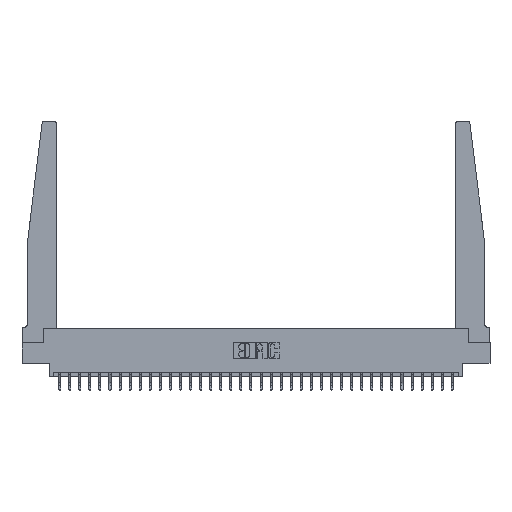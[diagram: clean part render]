
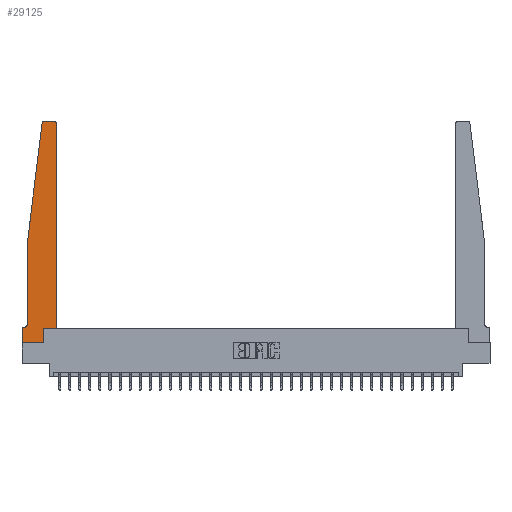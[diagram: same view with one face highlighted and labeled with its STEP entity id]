
A CAD part, top view. The second image highlights one B-rep face of the part: STEP entity #29125.
In plain terms, the highlighted planar face has unit normal (0, 0, 1).
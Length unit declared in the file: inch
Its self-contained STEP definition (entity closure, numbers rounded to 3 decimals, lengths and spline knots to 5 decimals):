
#101 = VERTEX_POINT ( 'NONE', #22427 ) ;
#402 = VERTEX_POINT ( 'NONE', #6686 ) ;
#504 = ORIENTED_EDGE ( 'NONE', *, *, #11489, .T. ) ;
#626 = VERTEX_POINT ( 'NONE', #10877 ) ;
#701 = AXIS2_PLACEMENT_3D ( 'NONE', #30100, #7908, #3069 ) ;
#1510 = DIRECTION ( 'NONE',  ( 1., 0., 0. ) ) ;
#1739 = DIRECTION ( 'NONE',  ( -1., 0., 0. ) ) ;
#1906 = LINE ( 'NONE', #29407, #7983 ) ;
#1941 = VERTEX_POINT ( 'NONE', #22807 ) ;
#2016 = AXIS2_PLACEMENT_3D ( 'NONE', #30453, #7793, #10555 ) ;
#2256 = EDGE_CURVE ( 'NONE', #402, #26183, #29090, .T. ) ;
#2539 = EDGE_CURVE ( 'NONE', #26183, #1941, #19875, .T. ) ;
#3069 = DIRECTION ( 'NONE',  ( -1., 0., 0. ) ) ;
#3505 = CARTESIAN_POINT ( 'NONE',  ( 0.2605, 0.18, 0.37 ) ) ;
#3759 = CARTESIAN_POINT ( 'NONE',  ( 0., 0., 0.37 ) ) ;
#3989 = ORIENTED_EDGE ( 'NONE', *, *, #30733, .T. ) ;
#4038 = ORIENTED_EDGE ( 'NONE', *, *, #2539, .T. ) ;
#4169 = VERTEX_POINT ( 'NONE', #20301 ) ;
#4777 = CARTESIAN_POINT ( 'NONE',  ( 0., 0., 0.37 ) ) ;
#5580 = ORIENTED_EDGE ( 'NONE', *, *, #31310, .T. ) ;
#5649 = LINE ( 'NONE', #10828, #10124 ) ;
#5750 = DIRECTION ( 'NONE',  ( 0., 0., 1. ) ) ;
#6127 = ORIENTED_EDGE ( 'NONE', *, *, #16061, .T. ) ;
#6518 = LINE ( 'NONE', #3759, #27397 ) ;
#6686 = CARTESIAN_POINT ( 'NONE',  ( 0.395, 2.75, 0.37 ) ) ;
#7451 = EDGE_CURVE ( 'NONE', #31533, #101, #13365, .T. ) ;
#7793 = DIRECTION ( 'NONE',  ( 0., 0., 1. ) ) ;
#7827 = FACE_OUTER_BOUND ( 'NONE', #25704, .T. ) ;
#7892 = CARTESIAN_POINT ( 'NONE',  ( 0.2605, 0., 0.37 ) ) ;
#7908 = DIRECTION ( 'NONE',  ( 0., 0., -1. ) ) ;
#7983 = VECTOR ( 'NONE', #11783, 39.37008 ) ;
#8486 = AXIS2_PLACEMENT_3D ( 'NONE', #18069, #5750, #23089 ) ;
#8631 = ORIENTED_EDGE ( 'NONE', *, *, #29438, .T. ) ;
#8646 = VECTOR ( 'NONE', #24227, 39.37008 ) ;
#9258 = AXIS2_PLACEMENT_3D ( 'NONE', #18044, #22742, #20772 ) ;
#9527 = VECTOR ( 'NONE', #17424, 39.37008 ) ;
#9723 = LINE ( 'NONE', #9867, #14755 ) ;
#9867 = CARTESIAN_POINT ( 'NONE',  ( 0.065, 1.25, 0.37 ) ) ;
#10124 = VECTOR ( 'NONE', #15526, 39.37008 ) ;
#10555 = DIRECTION ( 'NONE',  ( 1., 0., 0. ) ) ;
#10763 = ORIENTED_EDGE ( 'NONE', *, *, #12258, .T. ) ;
#10828 = CARTESIAN_POINT ( 'NONE',  ( 0.065, 0.1875, 0.37 ) ) ;
#10877 = CARTESIAN_POINT ( 'NONE',  ( 0., 0., 0.37 ) ) ;
#11275 = CARTESIAN_POINT ( 'NONE',  ( 0.065, 0.2375, 0.37 ) ) ;
#11489 = EDGE_CURVE ( 'NONE', #12859, #12520, #1906, .T. ) ;
#11535 = DIRECTION ( 'NONE',  ( 0., -1., 0. ) ) ;
#11783 = DIRECTION ( 'NONE',  ( 0., 1., 0. ) ) ;
#12258 = EDGE_CURVE ( 'NONE', #14881, #27483, #9723, .T. ) ;
#12520 = VERTEX_POINT ( 'NONE', #29776 ) ;
#12859 = VERTEX_POINT ( 'NONE', #26493 ) ;
#12861 = PLANE ( 'NONE',  #9258 ) ;
#13365 = LINE ( 'NONE', #3505, #21335 ) ;
#14755 = VECTOR ( 'NONE', #11535, 39.37008 ) ;
#14832 = LINE ( 'NONE', #16768, #8646 ) ;
#14881 = VERTEX_POINT ( 'NONE', #19073 ) ;
#15020 = VERTEX_POINT ( 'NONE', #23779 ) ;
#15302 = VECTOR ( 'NONE', #1739, 39.37008 ) ;
#15526 = DIRECTION ( 'NONE',  ( -1., 0., 0. ) ) ;
#16061 = EDGE_CURVE ( 'NONE', #27483, #4169, #21400, .T. ) ;
#16768 = CARTESIAN_POINT ( 'NONE',  ( 0.065, 1.25, 0.37 ) ) ;
#16770 = EDGE_CURVE ( 'NONE', #15020, #626, #31631, .T. ) ;
#17424 = DIRECTION ( 'NONE',  ( 0., -1., 0. ) ) ;
#17673 = ORIENTED_EDGE ( 'NONE', *, *, #7451, .T. ) ;
#18044 = CARTESIAN_POINT ( 'NONE',  ( 0., 0.1875, 0.37 ) ) ;
#18069 = CARTESIAN_POINT ( 'NONE',  ( 0.27653, 2.72, 0.37 ) ) ;
#18947 = CARTESIAN_POINT ( 'NONE',  ( 0.425, 0.18, 0.37 ) ) ;
#19073 = CARTESIAN_POINT ( 'NONE',  ( 0.065, 1.25, 0.37 ) ) ;
#19875 = CIRCLE ( 'NONE', #8486, 0.03 ) ;
#20205 = VECTOR ( 'NONE', #29302, 39.37008 ) ;
#20301 = CARTESIAN_POINT ( 'NONE',  ( 0.015, 0.1875, 0.37 ) ) ;
#20772 = DIRECTION ( 'NONE',  ( 1., 0., 0. ) ) ;
#21335 = VECTOR ( 'NONE', #23258, 39.37008 ) ;
#21400 = CIRCLE ( 'NONE', #701, 0.05 ) ;
#22427 = CARTESIAN_POINT ( 'NONE',  ( 0.2605, 0.18, 0.37 ) ) ;
#22742 = DIRECTION ( 'NONE',  ( 0., 0., 1. ) ) ;
#22807 = CARTESIAN_POINT ( 'NONE',  ( 0.24675, 2.72367, 0.37 ) ) ;
#23089 = DIRECTION ( 'NONE',  ( 1., 0., 0. ) ) ;
#23258 = DIRECTION ( 'NONE',  ( 0., 1., 0. ) ) ;
#23424 = EDGE_CURVE ( 'NONE', #4169, #15020, #5649, .T. ) ;
#23714 = ORIENTED_EDGE ( 'NONE', *, *, #16770, .T. ) ;
#23779 = CARTESIAN_POINT ( 'NONE',  ( 0., 0.1875, 0.37 ) ) ;
#23881 = CARTESIAN_POINT ( 'NONE',  ( 0.27653, 2.75, 0.37 ) ) ;
#23918 = CARTESIAN_POINT ( 'NONE',  ( 0.25, 2.75, 0.37 ) ) ;
#24227 = DIRECTION ( 'NONE',  ( -0.122, -0.992, 0. ) ) ;
#25580 = EDGE_CURVE ( 'NONE', #1941, #14881, #14832, .T. ) ;
#25704 = EDGE_LOOP ( 'NONE', ( #30868, #4038, #30411, #10763, #6127, #31049, #23714, #3989, #17673, #5580, #504, #8631 ) ) ;
#26183 = VERTEX_POINT ( 'NONE', #23881 ) ;
#26375 = LINE ( 'NONE', #18947, #20205 ) ;
#26493 = CARTESIAN_POINT ( 'NONE',  ( 0.425, 0.18, 0.37 ) ) ;
#26816 = CIRCLE ( 'NONE', #2016, 0.03 ) ;
#27397 = VECTOR ( 'NONE', #1510, 39.37008 ) ;
#27483 = VERTEX_POINT ( 'NONE', #11275 ) ;
#29090 = LINE ( 'NONE', #23918, #15302 ) ;
#29125 = ADVANCED_FACE ( 'NONE', ( #7827 ), #12861, .T. ) ;
#29302 = DIRECTION ( 'NONE',  ( 1., 0., 0. ) ) ;
#29407 = CARTESIAN_POINT ( 'NONE',  ( 0.425, 0.18, 0.37 ) ) ;
#29438 = EDGE_CURVE ( 'NONE', #12520, #402, #26816, .T. ) ;
#29776 = CARTESIAN_POINT ( 'NONE',  ( 0.425, 2.72, 0.37 ) ) ;
#30100 = CARTESIAN_POINT ( 'NONE',  ( 0.015, 0.2375, 0.37 ) ) ;
#30411 = ORIENTED_EDGE ( 'NONE', *, *, #25580, .T. ) ;
#30453 = CARTESIAN_POINT ( 'NONE',  ( 0.395, 2.72, 0.37 ) ) ;
#30733 = EDGE_CURVE ( 'NONE', #626, #31533, #6518, .T. ) ;
#30868 = ORIENTED_EDGE ( 'NONE', *, *, #2256, .T. ) ;
#31049 = ORIENTED_EDGE ( 'NONE', *, *, #23424, .T. ) ;
#31310 = EDGE_CURVE ( 'NONE', #101, #12859, #26375, .T. ) ;
#31533 = VERTEX_POINT ( 'NONE', #7892 ) ;
#31631 = LINE ( 'NONE', #4777, #9527 ) ;
